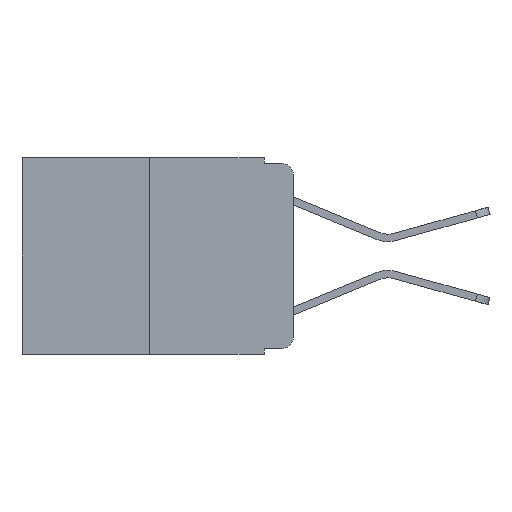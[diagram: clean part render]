
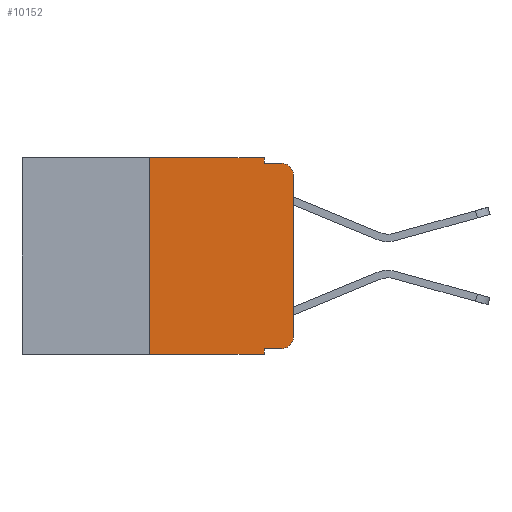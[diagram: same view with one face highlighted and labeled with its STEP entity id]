
A CAD part, left-side view. The second image highlights one B-rep face of the part: STEP entity #10152.
In plain terms, the highlighted planar face has unit normal (-1, 0, 0).
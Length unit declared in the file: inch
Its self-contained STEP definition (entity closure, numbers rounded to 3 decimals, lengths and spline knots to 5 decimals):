
#89 = CARTESIAN_POINT ( 'NONE',  ( 0., 0.051, 0. ) ) ;
#270 = EDGE_CURVE ( 'NONE', #2720, #8187, #9363, .T. ) ;
#502 = CARTESIAN_POINT ( 'NONE',  ( 0., 0.051, -0.333 ) ) ;
#550 = DIRECTION ( 'NONE',  ( 0., 0., -1. ) ) ;
#601 = EDGE_CURVE ( 'NONE', #5667, #10724, #4585, .T. ) ;
#660 = DIRECTION ( 'NONE',  ( 0., -1., 0. ) ) ;
#683 = VERTEX_POINT ( 'NONE', #6720 ) ;
#1283 = EDGE_CURVE ( 'NONE', #3364, #3651, #7287, .T. ) ;
#1366 = VERTEX_POINT ( 'NONE', #7994 ) ;
#1440 = DIRECTION ( 'NONE',  ( 0., 0., -1. ) ) ;
#1494 = AXIS2_PLACEMENT_3D ( 'NONE', #4232, #5219, #5901 ) ;
#2306 = CARTESIAN_POINT ( 'NONE',  ( 0., 0.25, 0. ) ) ;
#2313 = DIRECTION ( 'NONE',  ( 0., 0., 1. ) ) ;
#2432 = EDGE_CURVE ( 'NONE', #6561, #2720, #2835, .T. ) ;
#2620 = EDGE_LOOP ( 'NONE', ( #6586, #4539, #7126, #9445, #9715, #2969, #5666, #7958, #5047, #9651 ) ) ;
#2667 = AXIS2_PLACEMENT_3D ( 'NONE', #9439, #6888, #1440 ) ;
#2720 = VERTEX_POINT ( 'NONE', #2306 ) ;
#2835 = LINE ( 'NONE', #3879, #8519 ) ;
#2969 = ORIENTED_EDGE ( 'NONE', *, *, #2432, .F. ) ;
#3031 = CARTESIAN_POINT ( 'NONE',  ( 0., 0.473, 0. ) ) ;
#3281 = CARTESIAN_POINT ( 'NONE',  ( 0., 0., -0.313 ) ) ;
#3296 = EDGE_CURVE ( 'NONE', #1366, #5667, #8584, .T. ) ;
#3364 = VERTEX_POINT ( 'NONE', #9063 ) ;
#3612 = VECTOR ( 'NONE', #660, 39.37008 ) ;
#3651 = VERTEX_POINT ( 'NONE', #7457 ) ;
#3738 = DIRECTION ( 'NONE',  ( 0., 0., 1. ) ) ;
#3879 = CARTESIAN_POINT ( 'NONE',  ( 0., 0.25, 0. ) ) ;
#3884 = EDGE_CURVE ( 'NONE', #6561, #683, #11493, .T. ) ;
#4019 = DIRECTION ( 'NONE',  ( 0., -1., 0. ) ) ;
#4143 = EDGE_CURVE ( 'NONE', #10724, #3364, #4735, .T. ) ;
#4232 = CARTESIAN_POINT ( 'NONE',  ( 0., 0.02, -0.313 ) ) ;
#4524 = VECTOR ( 'NONE', #550, 39.37008 ) ;
#4534 = VECTOR ( 'NONE', #5479, 39.37008 ) ;
#4539 = ORIENTED_EDGE ( 'NONE', *, *, #1283, .T. ) ;
#4585 = CIRCLE ( 'NONE', #1494, 0.02 ) ;
#4661 = LINE ( 'NONE', #5828, #9029 ) ;
#4735 = LINE ( 'NONE', #6988, #10841 ) ;
#4828 = FACE_OUTER_BOUND ( 'NONE', #2620, .T. ) ;
#5047 = ORIENTED_EDGE ( 'NONE', *, *, #3296, .T. ) ;
#5098 = LINE ( 'NONE', #11272, #4524 ) ;
#5219 = DIRECTION ( 'NONE',  ( -1., 0., 0. ) ) ;
#5299 = CARTESIAN_POINT ( 'NONE',  ( 0., 0.02, -0.03 ) ) ;
#5436 = CARTESIAN_POINT ( 'NONE',  ( 0., 0.051, -0.01 ) ) ;
#5479 = DIRECTION ( 'NONE',  ( 0., -1., 0. ) ) ;
#5666 = ORIENTED_EDGE ( 'NONE', *, *, #3884, .T. ) ;
#5667 = VERTEX_POINT ( 'NONE', #6146 ) ;
#5828 = CARTESIAN_POINT ( 'NONE',  ( 0., 0.051, 0. ) ) ;
#5901 = DIRECTION ( 'NONE',  ( 0., 0., -1. ) ) ;
#6146 = CARTESIAN_POINT ( 'NONE',  ( 0., 0.02, -0.333 ) ) ;
#6338 = CARTESIAN_POINT ( 'NONE',  ( 0., 0.473, -0.343 ) ) ;
#6417 = EDGE_CURVE ( 'NONE', #7741, #3651, #6852, .T. ) ;
#6561 = VERTEX_POINT ( 'NONE', #10003 ) ;
#6586 = ORIENTED_EDGE ( 'NONE', *, *, #4143, .T. ) ;
#6630 = EDGE_CURVE ( 'NONE', #8187, #7741, #4661, .T. ) ;
#6662 = DIRECTION ( 'NONE',  ( 0., 0., -1. ) ) ;
#6720 = CARTESIAN_POINT ( 'NONE',  ( 0., 0.051, -0.343 ) ) ;
#6850 = EDGE_CURVE ( 'NONE', #1366, #683, #5098, .T. ) ;
#6852 = LINE ( 'NONE', #5436, #4534 ) ;
#6888 = DIRECTION ( 'NONE',  ( 1., 0., 0. ) ) ;
#6911 = VECTOR ( 'NONE', #8510, 39.37008 ) ;
#6988 = CARTESIAN_POINT ( 'NONE',  ( 0., 0., 0. ) ) ;
#7126 = ORIENTED_EDGE ( 'NONE', *, *, #6417, .F. ) ;
#7287 = CIRCLE ( 'NONE', #7724, 0.02 ) ;
#7457 = CARTESIAN_POINT ( 'NONE',  ( 0., 0.02, -0.01 ) ) ;
#7724 = AXIS2_PLACEMENT_3D ( 'NONE', #5299, #9762, #9617 ) ;
#7741 = VERTEX_POINT ( 'NONE', #10924 ) ;
#7958 = ORIENTED_EDGE ( 'NONE', *, *, #6850, .F. ) ;
#7994 = CARTESIAN_POINT ( 'NONE',  ( 0., 0.051, -0.333 ) ) ;
#8187 = VERTEX_POINT ( 'NONE', #89 ) ;
#8510 = DIRECTION ( 'NONE',  ( 0., -1., 0. ) ) ;
#8519 = VECTOR ( 'NONE', #3738, 39.37008 ) ;
#8584 = LINE ( 'NONE', #502, #3612 ) ;
#9029 = VECTOR ( 'NONE', #6662, 39.37008 ) ;
#9063 = CARTESIAN_POINT ( 'NONE',  ( 0., 0., -0.03 ) ) ;
#9363 = LINE ( 'NONE', #3031, #9893 ) ;
#9439 = CARTESIAN_POINT ( 'NONE',  ( 0., 0.473, 0. ) ) ;
#9445 = ORIENTED_EDGE ( 'NONE', *, *, #6630, .F. ) ;
#9617 = DIRECTION ( 'NONE',  ( 0., 0., -1. ) ) ;
#9651 = ORIENTED_EDGE ( 'NONE', *, *, #601, .T. ) ;
#9715 = ORIENTED_EDGE ( 'NONE', *, *, #270, .F. ) ;
#9762 = DIRECTION ( 'NONE',  ( -1., 0., 0. ) ) ;
#9893 = VECTOR ( 'NONE', #4019, 39.37008 ) ;
#10003 = CARTESIAN_POINT ( 'NONE',  ( 0., 0.25, -0.343 ) ) ;
#10152 = ADVANCED_FACE ( 'NONE', ( #4828 ), #10351, .F. ) ;
#10351 = PLANE ( 'NONE',  #2667 ) ;
#10724 = VERTEX_POINT ( 'NONE', #3281 ) ;
#10841 = VECTOR ( 'NONE', #2313, 39.37008 ) ;
#10924 = CARTESIAN_POINT ( 'NONE',  ( 0., 0.051, -0.01 ) ) ;
#11272 = CARTESIAN_POINT ( 'NONE',  ( 0., 0.051, 0. ) ) ;
#11493 = LINE ( 'NONE', #6338, #6911 ) ;
